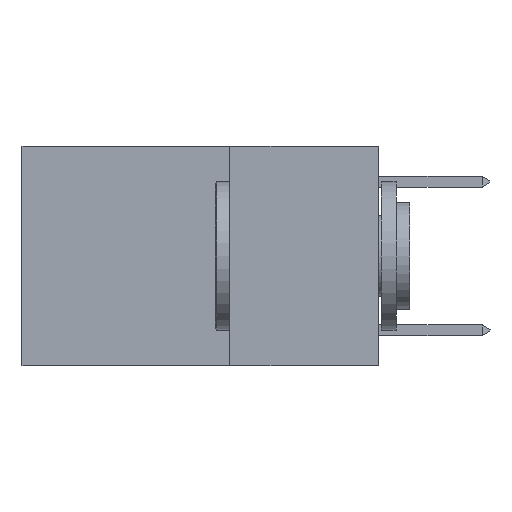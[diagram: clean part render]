
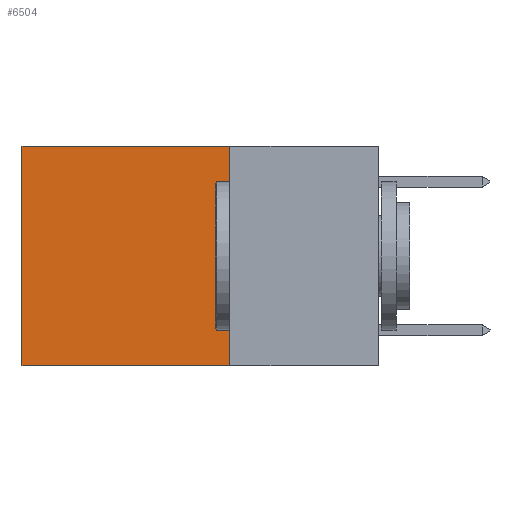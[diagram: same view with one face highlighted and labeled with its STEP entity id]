
A CAD part, left-side view. The second image highlights one B-rep face of the part: STEP entity #6504.
In plain terms, the highlighted planar face has unit normal (-1, 0, 0).
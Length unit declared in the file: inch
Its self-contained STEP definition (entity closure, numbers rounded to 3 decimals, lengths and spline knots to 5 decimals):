
#756 = ORIENTED_EDGE ( 'NONE', *, *, #13722, .T. ) ;
#1552 = DIRECTION ( 'NONE',  ( 0., 0., -1. ) ) ;
#2244 = CARTESIAN_POINT ( 'NONE',  ( 0.2625, 0.25, 0. ) ) ;
#2429 = VECTOR ( 'NONE', #15432, 39.37008 ) ;
#2520 = CARTESIAN_POINT ( 'NONE',  ( 0.2625, 0.6, 0. ) ) ;
#2732 = AXIS2_PLACEMENT_3D ( 'NONE', #7000, #7061, #16497 ) ;
#2751 = CARTESIAN_POINT ( 'NONE',  ( 0.2625, 0.25, -0.37 ) ) ;
#3804 = ORIENTED_EDGE ( 'NONE', *, *, #5424, .T. ) ;
#4917 = VERTEX_POINT ( 'NONE', #2244 ) ;
#5068 = FACE_OUTER_BOUND ( 'NONE', #16501, .T. ) ;
#5424 = EDGE_CURVE ( 'NONE', #16101, #16226, #13357, .T. ) ;
#5733 = LINE ( 'NONE', #13880, #15651 ) ;
#6504 = ADVANCED_FACE ( 'NONE', ( #5068 ), #9678, .F. ) ;
#6647 = CARTESIAN_POINT ( 'NONE',  ( 0.2625, 0.25, 0. ) ) ;
#6963 = VECTOR ( 'NONE', #10918, 39.37008 ) ;
#7000 = CARTESIAN_POINT ( 'NONE',  ( 0.2625, 0.25, 0. ) ) ;
#7061 = DIRECTION ( 'NONE',  ( 1., 0., 0. ) ) ;
#7434 = ORIENTED_EDGE ( 'NONE', *, *, #11173, .F. ) ;
#7850 = ORIENTED_EDGE ( 'NONE', *, *, #9809, .F. ) ;
#7995 = DIRECTION ( 'NONE',  ( 0., 1., 0. ) ) ;
#8357 = LINE ( 'NONE', #6647, #15130 ) ;
#9678 = PLANE ( 'NONE',  #2732 ) ;
#9809 = EDGE_CURVE ( 'NONE', #4917, #14054, #5733, .T. ) ;
#10918 = DIRECTION ( 'NONE',  ( 0., 1., 0. ) ) ;
#11173 = EDGE_CURVE ( 'NONE', #14054, #16226, #14114, .T. ) ;
#11224 = CARTESIAN_POINT ( 'NONE',  ( 0.2625, 0.6, 0. ) ) ;
#13357 = LINE ( 'NONE', #11224, #2429 ) ;
#13642 = CARTESIAN_POINT ( 'NONE',  ( 0.2625, 0.6, -0.37 ) ) ;
#13722 = EDGE_CURVE ( 'NONE', #4917, #16101, #8357, .T. ) ;
#13865 = CARTESIAN_POINT ( 'NONE',  ( 0.2625, 0.25, -0.37 ) ) ;
#13880 = CARTESIAN_POINT ( 'NONE',  ( 0.2625, 0.25, 0. ) ) ;
#14054 = VERTEX_POINT ( 'NONE', #13865 ) ;
#14114 = LINE ( 'NONE', #2751, #6963 ) ;
#15130 = VECTOR ( 'NONE', #7995, 39.37008 ) ;
#15432 = DIRECTION ( 'NONE',  ( 0., 0., -1. ) ) ;
#15651 = VECTOR ( 'NONE', #1552, 39.37008 ) ;
#16101 = VERTEX_POINT ( 'NONE', #2520 ) ;
#16226 = VERTEX_POINT ( 'NONE', #13642 ) ;
#16497 = DIRECTION ( 'NONE',  ( 0., 0., -1. ) ) ;
#16501 = EDGE_LOOP ( 'NONE', ( #3804, #7434, #7850, #756 ) ) ;
